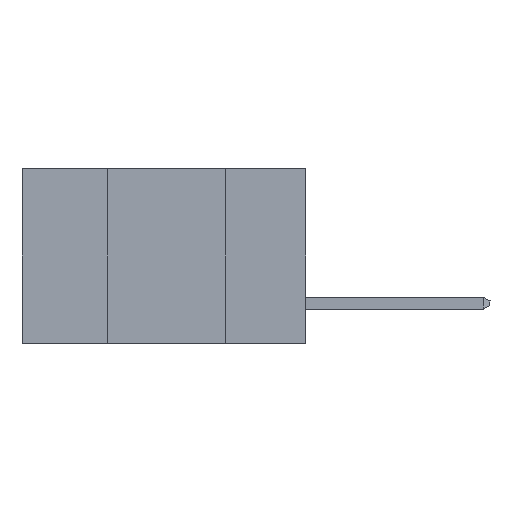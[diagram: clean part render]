
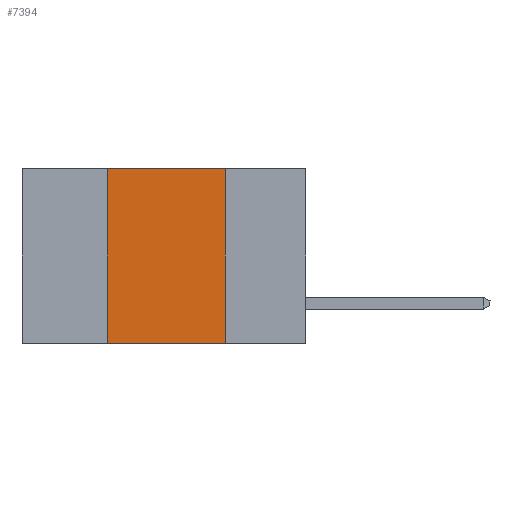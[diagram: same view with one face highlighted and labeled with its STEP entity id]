
A CAD part, left-side view. The second image highlights one B-rep face of the part: STEP entity #7394.
In plain terms, the highlighted planar face has unit normal (-1, 0, 0).
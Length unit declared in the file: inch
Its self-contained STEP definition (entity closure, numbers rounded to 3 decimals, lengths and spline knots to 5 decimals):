
#33 = EDGE_LOOP ( 'NONE', ( #16961, #19279, #9678, #15322 ) ) ;
#665 = DIRECTION ( 'NONE',  ( 0., -1., 0. ) ) ;
#732 = CARTESIAN_POINT ( 'NONE',  ( 0., 0.6, 0. ) ) ;
#892 = DIRECTION ( 'NONE',  ( 0., 0., -1. ) ) ;
#1092 = CARTESIAN_POINT ( 'NONE',  ( 0., 0.42, 0. ) ) ;
#2581 = CARTESIAN_POINT ( 'NONE',  ( 0., 0.6, -0.37 ) ) ;
#2798 = VECTOR ( 'NONE', #14302, 39.37008 ) ;
#2899 = EDGE_CURVE ( 'NONE', #16346, #11338, #16067, .T. ) ;
#4156 = VECTOR ( 'NONE', #4219, 39.37008 ) ;
#4219 = DIRECTION ( 'NONE',  ( 0., -1., 0. ) ) ;
#4364 = VECTOR ( 'NONE', #18038, 39.37008 ) ;
#5227 = VERTEX_POINT ( 'NONE', #15599 ) ;
#5540 = VECTOR ( 'NONE', #665, 39.37008 ) ;
#5593 = CARTESIAN_POINT ( 'NONE',  ( 0., 0.6, 0. ) ) ;
#7299 = FACE_OUTER_BOUND ( 'NONE', #33, .T. ) ;
#7394 = ADVANCED_FACE ( 'NONE', ( #7299 ), #18876, .F. ) ;
#7689 = EDGE_CURVE ( 'NONE', #16346, #5227, #8573, .T. ) ;
#8358 = CARTESIAN_POINT ( 'NONE',  ( 0., 0.17, 0. ) ) ;
#8573 = LINE ( 'NONE', #2581, #4156 ) ;
#8779 = LINE ( 'NONE', #14722, #4364 ) ;
#8781 = VERTEX_POINT ( 'NONE', #8358 ) ;
#8787 = CARTESIAN_POINT ( 'NONE',  ( 0., 0.42, 0. ) ) ;
#9678 = ORIENTED_EDGE ( 'NONE', *, *, #2899, .F. ) ;
#10897 = CARTESIAN_POINT ( 'NONE',  ( 0., 0.42, -0.37 ) ) ;
#11338 = VERTEX_POINT ( 'NONE', #8787 ) ;
#12071 = LINE ( 'NONE', #732, #5540 ) ;
#14085 = DIRECTION ( 'NONE',  ( 1., 0., 0. ) ) ;
#14302 = DIRECTION ( 'NONE',  ( 0., 0., 1. ) ) ;
#14722 = CARTESIAN_POINT ( 'NONE',  ( 0., 0.17, 0. ) ) ;
#15322 = ORIENTED_EDGE ( 'NONE', *, *, #7689, .T. ) ;
#15599 = CARTESIAN_POINT ( 'NONE',  ( 0., 0.17, -0.37 ) ) ;
#16067 = LINE ( 'NONE', #1092, #2798 ) ;
#16346 = VERTEX_POINT ( 'NONE', #10897 ) ;
#16529 = EDGE_CURVE ( 'NONE', #8781, #5227, #8779, .T. ) ;
#16961 = ORIENTED_EDGE ( 'NONE', *, *, #16529, .F. ) ;
#18038 = DIRECTION ( 'NONE',  ( 0., 0., -1. ) ) ;
#18790 = EDGE_CURVE ( 'NONE', #11338, #8781, #12071, .T. ) ;
#18876 = PLANE ( 'NONE',  #19462 ) ;
#19279 = ORIENTED_EDGE ( 'NONE', *, *, #18790, .F. ) ;
#19462 = AXIS2_PLACEMENT_3D ( 'NONE', #5593, #14085, #892 ) ;
